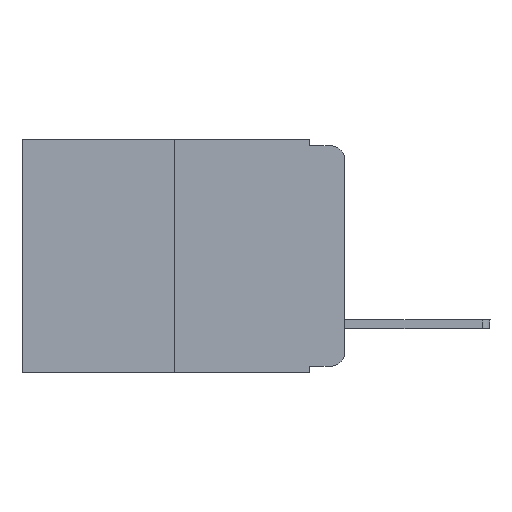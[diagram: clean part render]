
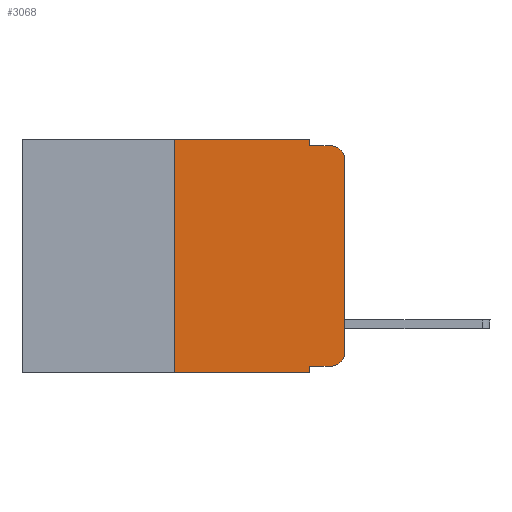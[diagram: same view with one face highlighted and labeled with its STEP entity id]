
A CAD part, left-side view. The second image highlights one B-rep face of the part: STEP entity #3068.
In plain terms, the highlighted planar face has unit normal (-1, 0, 0).
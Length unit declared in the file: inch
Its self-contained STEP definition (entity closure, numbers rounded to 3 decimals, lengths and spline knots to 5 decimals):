
#102 = VECTOR ( 'NONE', #6845, 39.37008 ) ;
#111 = FACE_OUTER_BOUND ( 'NONE', #7827, .T. ) ;
#320 = CARTESIAN_POINT ( 'NONE',  ( 0., 0.051, -0.333 ) ) ;
#375 = CARTESIAN_POINT ( 'NONE',  ( 0., 0.473, 0. ) ) ;
#513 = AXIS2_PLACEMENT_3D ( 'NONE', #1755, #4320, #8044 ) ;
#545 = ORIENTED_EDGE ( 'NONE', *, *, #6839, .T. ) ;
#624 = ORIENTED_EDGE ( 'NONE', *, *, #3175, .T. ) ;
#635 = AXIS2_PLACEMENT_3D ( 'NONE', #8107, #5014, #7969 ) ;
#726 = DIRECTION ( 'NONE',  ( 0., 0., -1. ) ) ;
#729 = VECTOR ( 'NONE', #8324, 39.37008 ) ;
#784 = CARTESIAN_POINT ( 'NONE',  ( 0., 0.051, -0.01 ) ) ;
#915 = ORIENTED_EDGE ( 'NONE', *, *, #8200, .T. ) ;
#1199 = LINE ( 'NONE', #3145, #729 ) ;
#1499 = DIRECTION ( 'NONE',  ( 0., -1., 0. ) ) ;
#1755 = CARTESIAN_POINT ( 'NONE',  ( 0., 0.02, -0.313 ) ) ;
#2015 = LINE ( 'NONE', #320, #5231 ) ;
#2205 = VERTEX_POINT ( 'NONE', #6437 ) ;
#2239 = CARTESIAN_POINT ( 'NONE',  ( 0., 0.473, -0.343 ) ) ;
#2339 = ORIENTED_EDGE ( 'NONE', *, *, #5340, .F. ) ;
#2432 = VERTEX_POINT ( 'NONE', #4355 ) ;
#2441 = VERTEX_POINT ( 'NONE', #8771 ) ;
#2550 = LINE ( 'NONE', #375, #102 ) ;
#2686 = VERTEX_POINT ( 'NONE', #4038 ) ;
#2807 = CARTESIAN_POINT ( 'NONE',  ( 0., 0.051, 0. ) ) ;
#2808 = ORIENTED_EDGE ( 'NONE', *, *, #3835, .F. ) ;
#2864 = LINE ( 'NONE', #784, #6216 ) ;
#2885 = CARTESIAN_POINT ( 'NONE',  ( 0., 0., 0. ) ) ;
#3013 = VERTEX_POINT ( 'NONE', #5918 ) ;
#3027 = EDGE_CURVE ( 'NONE', #3452, #7942, #6940, .T. ) ;
#3068 = ADVANCED_FACE ( 'NONE', ( #111 ), #8111, .F. ) ;
#3145 = CARTESIAN_POINT ( 'NONE',  ( 0., 0.051, 0. ) ) ;
#3175 = EDGE_CURVE ( 'NONE', #2432, #2686, #5182, .T. ) ;
#3452 = VERTEX_POINT ( 'NONE', #4268 ) ;
#3661 = CARTESIAN_POINT ( 'NONE',  ( 0., 0.473, 0. ) ) ;
#3812 = VECTOR ( 'NONE', #8766, 39.37008 ) ;
#3835 = EDGE_CURVE ( 'NONE', #9151, #4027, #2550, .T. ) ;
#3993 = CARTESIAN_POINT ( 'NONE',  ( 0., 0.051, -0.333 ) ) ;
#4027 = VERTEX_POINT ( 'NONE', #2807 ) ;
#4038 = CARTESIAN_POINT ( 'NONE',  ( 0., 0.02, -0.01 ) ) ;
#4198 = EDGE_CURVE ( 'NONE', #3013, #2686, #2864, .T. ) ;
#4224 = AXIS2_PLACEMENT_3D ( 'NONE', #3661, #5894, #5662 ) ;
#4227 = LINE ( 'NONE', #2239, #8627 ) ;
#4268 = CARTESIAN_POINT ( 'NONE',  ( 0., 0.02, -0.333 ) ) ;
#4320 = DIRECTION ( 'NONE',  ( -1., 0., 0. ) ) ;
#4355 = CARTESIAN_POINT ( 'NONE',  ( 0., 0., -0.03 ) ) ;
#4552 = ORIENTED_EDGE ( 'NONE', *, *, #4198, .F. ) ;
#5014 = DIRECTION ( 'NONE',  ( -1., 0., 0. ) ) ;
#5098 = EDGE_CURVE ( 'NONE', #8963, #3452, #2015, .T. ) ;
#5182 = CIRCLE ( 'NONE', #635, 0.02 ) ;
#5231 = VECTOR ( 'NONE', #8486, 39.37008 ) ;
#5277 = LINE ( 'NONE', #2885, #8527 ) ;
#5340 = EDGE_CURVE ( 'NONE', #2205, #9151, #8224, .T. ) ;
#5662 = DIRECTION ( 'NONE',  ( 0., 0., -1. ) ) ;
#5894 = DIRECTION ( 'NONE',  ( 1., 0., 0. ) ) ;
#5918 = CARTESIAN_POINT ( 'NONE',  ( 0., 0.051, -0.01 ) ) ;
#6114 = ORIENTED_EDGE ( 'NONE', *, *, #9480, .F. ) ;
#6216 = VECTOR ( 'NONE', #1499, 39.37008 ) ;
#6305 = ORIENTED_EDGE ( 'NONE', *, *, #7527, .F. ) ;
#6378 = CARTESIAN_POINT ( 'NONE',  ( 0., 0.25, 0. ) ) ;
#6437 = CARTESIAN_POINT ( 'NONE',  ( 0., 0.25, -0.343 ) ) ;
#6781 = LINE ( 'NONE', #9510, #7614 ) ;
#6839 = EDGE_CURVE ( 'NONE', #7942, #2432, #5277, .T. ) ;
#6845 = DIRECTION ( 'NONE',  ( 0., -1., 0. ) ) ;
#6865 = DIRECTION ( 'NONE',  ( 0., -1., 0. ) ) ;
#6940 = CIRCLE ( 'NONE', #513, 0.02 ) ;
#7474 = ORIENTED_EDGE ( 'NONE', *, *, #3027, .T. ) ;
#7527 = EDGE_CURVE ( 'NONE', #8963, #2441, #6781, .T. ) ;
#7614 = VECTOR ( 'NONE', #726, 39.37008 ) ;
#7827 = EDGE_LOOP ( 'NONE', ( #545, #624, #4552, #6114, #2808, #2339, #915, #6305, #8587, #7474 ) ) ;
#7942 = VERTEX_POINT ( 'NONE', #9464 ) ;
#7969 = DIRECTION ( 'NONE',  ( 0., 0., -1. ) ) ;
#8006 = CARTESIAN_POINT ( 'NONE',  ( 0., 0.25, 0. ) ) ;
#8044 = DIRECTION ( 'NONE',  ( 0., 0., -1. ) ) ;
#8087 = DIRECTION ( 'NONE',  ( 0., 0., 1. ) ) ;
#8107 = CARTESIAN_POINT ( 'NONE',  ( 0., 0.02, -0.03 ) ) ;
#8111 = PLANE ( 'NONE',  #4224 ) ;
#8200 = EDGE_CURVE ( 'NONE', #2205, #2441, #4227, .T. ) ;
#8224 = LINE ( 'NONE', #8006, #3812 ) ;
#8324 = DIRECTION ( 'NONE',  ( 0., 0., -1. ) ) ;
#8486 = DIRECTION ( 'NONE',  ( 0., -1., 0. ) ) ;
#8527 = VECTOR ( 'NONE', #8087, 39.37008 ) ;
#8587 = ORIENTED_EDGE ( 'NONE', *, *, #5098, .T. ) ;
#8627 = VECTOR ( 'NONE', #6865, 39.37008 ) ;
#8766 = DIRECTION ( 'NONE',  ( 0., 0., 1. ) ) ;
#8771 = CARTESIAN_POINT ( 'NONE',  ( 0., 0.051, -0.343 ) ) ;
#8963 = VERTEX_POINT ( 'NONE', #3993 ) ;
#9151 = VERTEX_POINT ( 'NONE', #6378 ) ;
#9464 = CARTESIAN_POINT ( 'NONE',  ( 0., 0., -0.313 ) ) ;
#9480 = EDGE_CURVE ( 'NONE', #4027, #3013, #1199, .T. ) ;
#9510 = CARTESIAN_POINT ( 'NONE',  ( 0., 0.051, 0. ) ) ;
